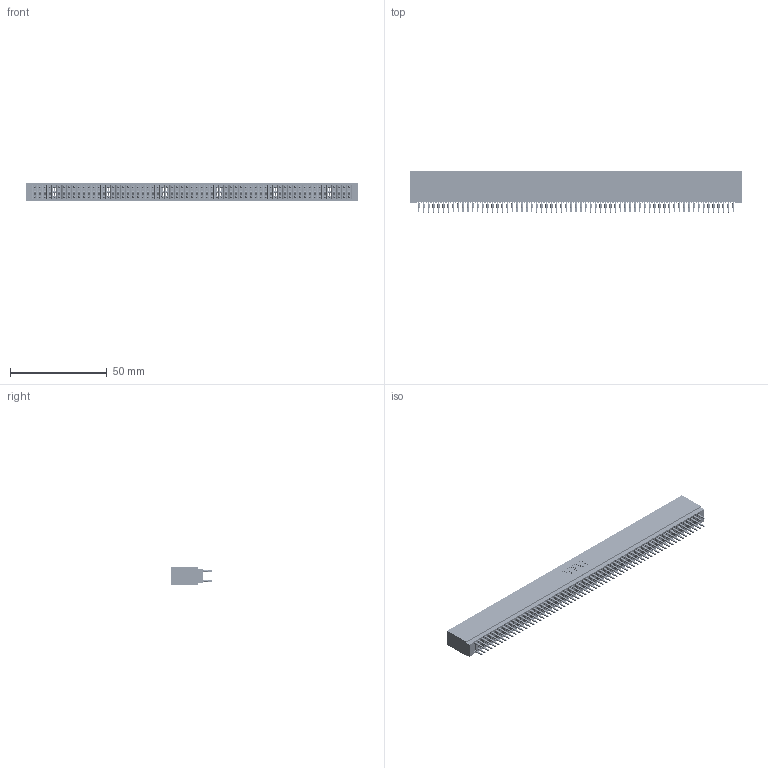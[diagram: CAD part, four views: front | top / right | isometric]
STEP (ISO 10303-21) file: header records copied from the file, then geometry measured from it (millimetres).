
FILE_DESCRIPTION (( 'STEP AP203' ), '1' );
FILE_NAME ('745-130-560-201.STEP', '2020-09-14T19:29:22', ( '' ), ( '' ), 'SwSTEP 2.0', 'SolidWorks 2020', '' );
FILE_SCHEMA (( 'CONFIG_CONTROL_DESIGN' ));
Length unit declared in the file: inch
Products named in the file (3): 745-292-001_560; 745 Part_Insulator Option - 01; 745-130-560-201
Assembly tree (131 placements, depth 2):
  745-130-560-201
    745 Part_Insulator Option - 01
    745-292-001_560  x130
Bounding box: 171.7 x 21.22 x 8.89 mm (x, y, z)
Volume: 15805.4 mm3; surface area: 34713.8 mm2
Topology: 131 solids, 131 shells, 12900 faces, 35293 edges, 22402 vertices
Faces by surface type: plane 6685, cylinder 2835, bspline 2600, torus 780
Entity records: 106618 total; most frequent: CARTESIAN_POINT 18989, ORIENTED_EDGE 18470, DIRECTION 16119, EDGE_CURVE 9235, LINE 8655, VECTOR 8655, VERTEX_POINT 5890, AXIS2_PLACEMENT_3D 3732
